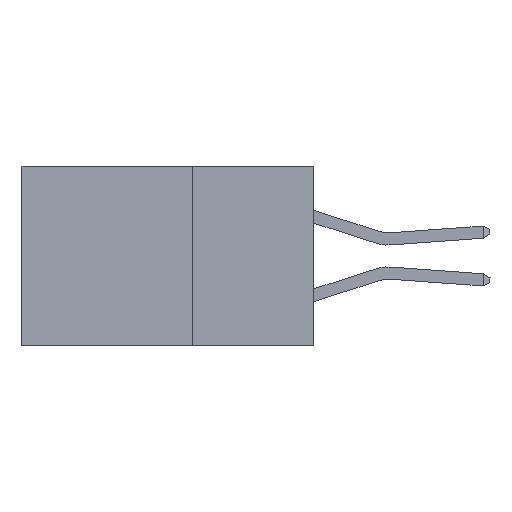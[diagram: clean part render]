
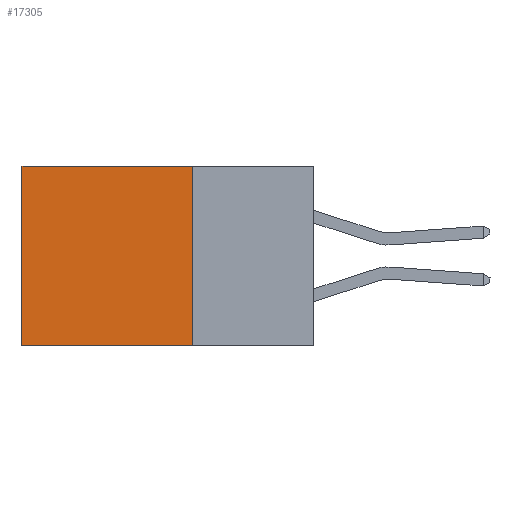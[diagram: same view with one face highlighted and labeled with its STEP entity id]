
A CAD part, left-side view. The second image highlights one B-rep face of the part: STEP entity #17305.
In plain terms, the highlighted planar face has unit normal (-1, 0, 0).
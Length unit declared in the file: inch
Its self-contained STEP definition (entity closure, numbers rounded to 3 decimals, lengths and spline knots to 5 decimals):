
#344 = PLANE ( 'NONE',  #16436 ) ;
#719 = CARTESIAN_POINT ( 'NONE',  ( 0.2875, 0.25, 0. ) ) ;
#730 = CARTESIAN_POINT ( 'NONE',  ( 0.2875, 0.6, 0. ) ) ;
#1170 = CARTESIAN_POINT ( 'NONE',  ( 0.2875, 0.6, -0.37 ) ) ;
#3318 = VERTEX_POINT ( 'NONE', #719 ) ;
#3682 = DIRECTION ( 'NONE',  ( 0., 1., 0. ) ) ;
#3822 = CARTESIAN_POINT ( 'NONE',  ( 0.2875, 0.6, 0. ) ) ;
#4197 = LINE ( 'NONE', #11408, #7852 ) ;
#4355 = ORIENTED_EDGE ( 'NONE', *, *, #5743, .F. ) ;
#4477 = VERTEX_POINT ( 'NONE', #5181 ) ;
#4503 = EDGE_CURVE ( 'NONE', #3318, #8907, #4197, .T. ) ;
#5132 = DIRECTION ( 'NONE',  ( 0., 0., -1. ) ) ;
#5181 = CARTESIAN_POINT ( 'NONE',  ( 0.2875, 0.25, -0.37 ) ) ;
#5347 = ORIENTED_EDGE ( 'NONE', *, *, #4503, .T. ) ;
#5383 = DIRECTION ( 'NONE',  ( 0., 0., -1. ) ) ;
#5743 = EDGE_CURVE ( 'NONE', #3318, #4477, #6577, .T. ) ;
#6577 = LINE ( 'NONE', #8586, #17808 ) ;
#6808 = CARTESIAN_POINT ( 'NONE',  ( 0.2875, 0.25, -0.37 ) ) ;
#7230 = ORIENTED_EDGE ( 'NONE', *, *, #15847, .T. ) ;
#7852 = VECTOR ( 'NONE', #3682, 39.37008 ) ;
#8586 = CARTESIAN_POINT ( 'NONE',  ( 0.2875, 0.25, 0. ) ) ;
#8907 = VERTEX_POINT ( 'NONE', #730 ) ;
#9747 = CARTESIAN_POINT ( 'NONE',  ( 0.2875, 0.25, 0. ) ) ;
#10111 = EDGE_CURVE ( 'NONE', #4477, #10394, #14392, .T. ) ;
#10394 = VERTEX_POINT ( 'NONE', #1170 ) ;
#10935 = FACE_OUTER_BOUND ( 'NONE', #18963, .T. ) ;
#11408 = CARTESIAN_POINT ( 'NONE',  ( 0.2875, 0.25, 0. ) ) ;
#11608 = DIRECTION ( 'NONE',  ( 0., 0., -1. ) ) ;
#11808 = LINE ( 'NONE', #3822, #19346 ) ;
#11965 = ORIENTED_EDGE ( 'NONE', *, *, #10111, .F. ) ;
#14382 = DIRECTION ( 'NONE',  ( 1., 0., 0. ) ) ;
#14392 = LINE ( 'NONE', #6808, #18349 ) ;
#14504 = DIRECTION ( 'NONE',  ( 0., 1., 0. ) ) ;
#15847 = EDGE_CURVE ( 'NONE', #8907, #10394, #11808, .T. ) ;
#16436 = AXIS2_PLACEMENT_3D ( 'NONE', #9747, #14382, #5132 ) ;
#17305 = ADVANCED_FACE ( 'NONE', ( #10935 ), #344, .F. ) ;
#17808 = VECTOR ( 'NONE', #11608, 39.37008 ) ;
#18349 = VECTOR ( 'NONE', #14504, 39.37008 ) ;
#18963 = EDGE_LOOP ( 'NONE', ( #7230, #11965, #4355, #5347 ) ) ;
#19346 = VECTOR ( 'NONE', #5383, 39.37008 ) ;
